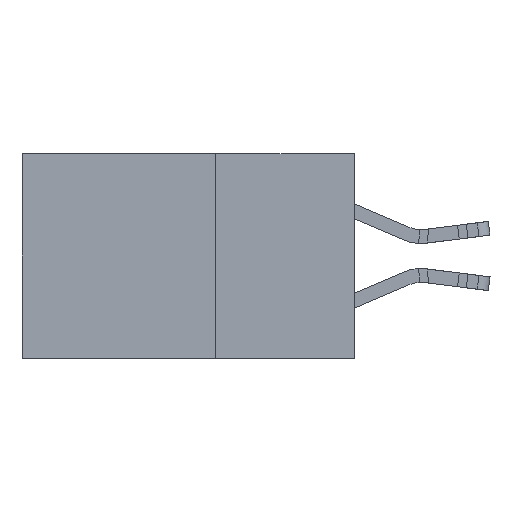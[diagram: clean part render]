
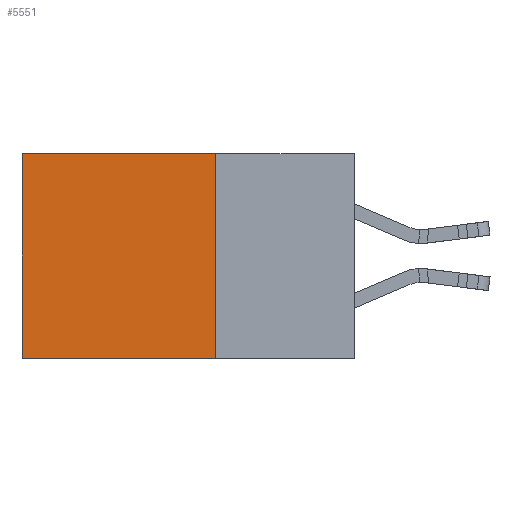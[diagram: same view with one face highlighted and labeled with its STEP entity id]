
A CAD part, left-side view. The second image highlights one B-rep face of the part: STEP entity #5551.
In plain terms, the highlighted planar face has unit normal (-1, 0, 0).
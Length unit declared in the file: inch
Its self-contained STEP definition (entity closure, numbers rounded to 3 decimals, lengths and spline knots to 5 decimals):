
#712 = CARTESIAN_POINT ( 'NONE',  ( 0.298, 0.6, 0. ) ) ;
#1189 = ORIENTED_EDGE ( 'NONE', *, *, #22990, .T. ) ;
#1992 = VERTEX_POINT ( 'NONE', #13670 ) ;
#2321 = LINE ( 'NONE', #21683, #33803 ) ;
#4500 = CARTESIAN_POINT ( 'NONE',  ( 0.298, 0.25, 0. ) ) ;
#4910 = LINE ( 'NONE', #13438, #31720 ) ;
#5196 = CARTESIAN_POINT ( 'NONE',  ( 0.298, 0.6, 0. ) ) ;
#5551 = ADVANCED_FACE ( 'NONE', ( #5854 ), #34618, .F. ) ;
#5854 = FACE_OUTER_BOUND ( 'NONE', #9292, .T. ) ;
#6320 = CARTESIAN_POINT ( 'NONE',  ( 0.298, 0.25, -0.37 ) ) ;
#6645 = VECTOR ( 'NONE', #12277, 39.37008 ) ;
#7458 = LINE ( 'NONE', #4500, #6645 ) ;
#8355 = DIRECTION ( 'NONE',  ( 0., 0., -1. ) ) ;
#8572 = EDGE_CURVE ( 'NONE', #18887, #1992, #26946, .T. ) ;
#8952 = ORIENTED_EDGE ( 'NONE', *, *, #19306, .F. ) ;
#9292 = EDGE_LOOP ( 'NONE', ( #29214, #8952, #30960, #1189 ) ) ;
#11427 = DIRECTION ( 'NONE',  ( 0., 0., -1. ) ) ;
#12277 = DIRECTION ( 'NONE',  ( 0., 1., 0. ) ) ;
#13438 = CARTESIAN_POINT ( 'NONE',  ( 0.298, 0.25, -0.37 ) ) ;
#13504 = VERTEX_POINT ( 'NONE', #6320 ) ;
#13670 = CARTESIAN_POINT ( 'NONE',  ( 0.298, 0.6, -0.37 ) ) ;
#13859 = EDGE_CURVE ( 'NONE', #28591, #13504, #2321, .T. ) ;
#17388 = AXIS2_PLACEMENT_3D ( 'NONE', #26321, #18510, #18735 ) ;
#18510 = DIRECTION ( 'NONE',  ( 1., 0., 0. ) ) ;
#18735 = DIRECTION ( 'NONE',  ( 0., 0., -1. ) ) ;
#18887 = VERTEX_POINT ( 'NONE', #712 ) ;
#19306 = EDGE_CURVE ( 'NONE', #13504, #1992, #4910, .T. ) ;
#21683 = CARTESIAN_POINT ( 'NONE',  ( 0.298, 0.25, 0. ) ) ;
#22286 = CARTESIAN_POINT ( 'NONE',  ( 0.298, 0.25, 0. ) ) ;
#22765 = VECTOR ( 'NONE', #8355, 39.37008 ) ;
#22990 = EDGE_CURVE ( 'NONE', #28591, #18887, #7458, .T. ) ;
#23799 = DIRECTION ( 'NONE',  ( 0., 1., 0. ) ) ;
#26321 = CARTESIAN_POINT ( 'NONE',  ( 0.298, 0.25, 0. ) ) ;
#26946 = LINE ( 'NONE', #5196, #22765 ) ;
#28591 = VERTEX_POINT ( 'NONE', #22286 ) ;
#29214 = ORIENTED_EDGE ( 'NONE', *, *, #8572, .T. ) ;
#30960 = ORIENTED_EDGE ( 'NONE', *, *, #13859, .F. ) ;
#31720 = VECTOR ( 'NONE', #23799, 39.37008 ) ;
#33803 = VECTOR ( 'NONE', #11427, 39.37008 ) ;
#34618 = PLANE ( 'NONE',  #17388 ) ;
